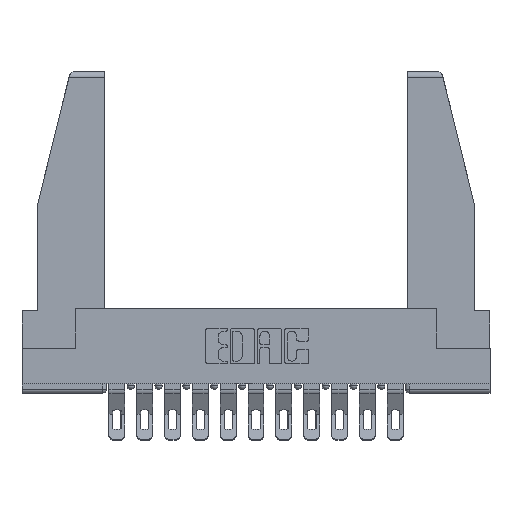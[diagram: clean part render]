
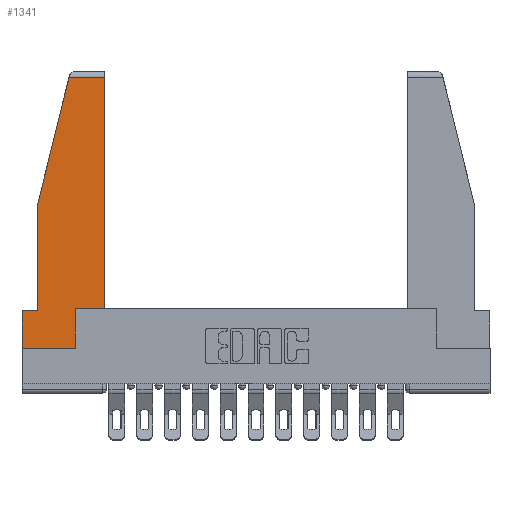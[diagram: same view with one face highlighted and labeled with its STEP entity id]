
A CAD part, top view. The second image highlights one B-rep face of the part: STEP entity #1341.
In plain terms, the highlighted planar face has unit normal (0, 0, 1).
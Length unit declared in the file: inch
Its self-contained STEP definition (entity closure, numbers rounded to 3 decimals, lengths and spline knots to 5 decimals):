
#149 = VERTEX_POINT ( 'NONE', #8627 ) ;
#550 = VERTEX_POINT ( 'NONE', #12458 ) ;
#1341 = ADVANCED_FACE ( 'NONE', ( #1440 ), #10790, .T. ) ;
#1440 = FACE_OUTER_BOUND ( 'NONE', #13769, .T. ) ;
#1858 = DIRECTION ( 'NONE',  ( 0., 0., 1. ) ) ;
#1907 = LINE ( 'NONE', #5243, #12119 ) ;
#2418 = CARTESIAN_POINT ( 'NONE',  ( 0.297, 0., 0. ) ) ;
#3054 = VECTOR ( 'NONE', #14526, 39.37008 ) ;
#3106 = CARTESIAN_POINT ( 'NONE',  ( 0., 0., 0. ) ) ;
#3108 = EDGE_CURVE ( 'NONE', #14425, #3875, #11947, .T. ) ;
#3682 = EDGE_CURVE ( 'NONE', #11848, #14425, #14760, .T. ) ;
#3747 = EDGE_CURVE ( 'NONE', #6221, #11848, #1907, .T. ) ;
#3875 = VERTEX_POINT ( 'NONE', #8193 ) ;
#3944 = EDGE_CURVE ( 'NONE', #13791, #149, #13099, .T. ) ;
#4106 = ORIENTED_EDGE ( 'NONE', *, *, #13910, .T. ) ;
#4577 = CARTESIAN_POINT ( 'NONE',  ( 0.297, 0.223, 0. ) ) ;
#5243 = CARTESIAN_POINT ( 'NONE',  ( 0., 0., 0. ) ) ;
#5554 = LINE ( 'NONE', #12822, #11363 ) ;
#5610 = AXIS2_PLACEMENT_3D ( 'NONE', #3106, #1858, #9544 ) ;
#6158 = VECTOR ( 'NONE', #15853, 39.37008 ) ;
#6221 = VERTEX_POINT ( 'NONE', #10349 ) ;
#6390 = LINE ( 'NONE', #9293, #8972 ) ;
#6427 = CARTESIAN_POINT ( 'NONE',  ( 0.297, 0., 0. ) ) ;
#6461 = ORIENTED_EDGE ( 'NONE', *, *, #3944, .T. ) ;
#6465 = CARTESIAN_POINT ( 'NONE',  ( 0.086, 0.21, 0. ) ) ;
#6560 = VECTOR ( 'NONE', #11701, 39.37008 ) ;
#6715 = VERTEX_POINT ( 'NONE', #11391 ) ;
#7686 = CARTESIAN_POINT ( 'NONE',  ( 0.297, 0.223, 0. ) ) ;
#7864 = DIRECTION ( 'NONE',  ( 1., 0., 0. ) ) ;
#7942 = ORIENTED_EDGE ( 'NONE', *, *, #13602, .T. ) ;
#8193 = CARTESIAN_POINT ( 'NONE',  ( 0.461, 0.223, 0. ) ) ;
#8423 = ORIENTED_EDGE ( 'NONE', *, *, #3682, .T. ) ;
#8551 = EDGE_CURVE ( 'NONE', #149, #550, #5554, .T. ) ;
#8627 = CARTESIAN_POINT ( 'NONE',  ( 0.2636, 1.52, 0. ) ) ;
#8797 = DIRECTION ( 'NONE',  ( 0., 1., 0. ) ) ;
#8857 = DIRECTION ( 'NONE',  ( 1., 0., 0. ) ) ;
#8949 = VECTOR ( 'NONE', #10043, 39.37008 ) ;
#8972 = VECTOR ( 'NONE', #9453, 39.37008 ) ;
#9088 = EDGE_CURVE ( 'NONE', #550, #14053, #11919, .T. ) ;
#9293 = CARTESIAN_POINT ( 'NONE',  ( 0., 0.21, 0. ) ) ;
#9453 = DIRECTION ( 'NONE',  ( -1., 0., 0. ) ) ;
#9478 = CARTESIAN_POINT ( 'NONE',  ( 0., 0.21, 0. ) ) ;
#9544 = DIRECTION ( 'NONE',  ( 1., 0., 0. ) ) ;
#9635 = ORIENTED_EDGE ( 'NONE', *, *, #3108, .T. ) ;
#9905 = CARTESIAN_POINT ( 'NONE',  ( 0.461, 0.223, 0. ) ) ;
#10043 = DIRECTION ( 'NONE',  ( 0., 1., 0. ) ) ;
#10349 = CARTESIAN_POINT ( 'NONE',  ( 0., 0., 0. ) ) ;
#10686 = EDGE_CURVE ( 'NONE', #6715, #6221, #15486, .T. ) ;
#10790 = PLANE ( 'NONE',  #5610 ) ;
#10803 = ORIENTED_EDGE ( 'NONE', *, *, #9088, .T. ) ;
#11363 = VECTOR ( 'NONE', #14133, 39.37008 ) ;
#11391 = CARTESIAN_POINT ( 'NONE',  ( 0., 0.21, 0. ) ) ;
#11571 = VECTOR ( 'NONE', #8857, 39.37008 ) ;
#11701 = DIRECTION ( 'NONE',  ( 0., -1., 0. ) ) ;
#11778 = ORIENTED_EDGE ( 'NONE', *, *, #10686, .T. ) ;
#11848 = VERTEX_POINT ( 'NONE', #6427 ) ;
#11911 = ORIENTED_EDGE ( 'NONE', *, *, #8551, .T. ) ;
#11919 = LINE ( 'NONE', #14325, #6560 ) ;
#11947 = LINE ( 'NONE', #7686, #11571 ) ;
#12119 = VECTOR ( 'NONE', #7864, 39.37008 ) ;
#12458 = CARTESIAN_POINT ( 'NONE',  ( 0.086, 0.8, 0. ) ) ;
#12822 = CARTESIAN_POINT ( 'NONE',  ( 0.271, 1.55, 0. ) ) ;
#13099 = LINE ( 'NONE', #14560, #6158 ) ;
#13337 = VECTOR ( 'NONE', #8797, 39.37008 ) ;
#13602 = EDGE_CURVE ( 'NONE', #14053, #6715, #6390, .T. ) ;
#13769 = EDGE_LOOP ( 'NONE', ( #4106, #6461, #11911, #10803, #7942, #11778, #14488, #8423, #9635 ) ) ;
#13791 = VERTEX_POINT ( 'NONE', #16010 ) ;
#13910 = EDGE_CURVE ( 'NONE', #3875, #13791, #14993, .T. ) ;
#14053 = VERTEX_POINT ( 'NONE', #6465 ) ;
#14133 = DIRECTION ( 'NONE',  ( -0.239, -0.971, 0. ) ) ;
#14325 = CARTESIAN_POINT ( 'NONE',  ( 0.086, 0.8, 0. ) ) ;
#14425 = VERTEX_POINT ( 'NONE', #4577 ) ;
#14488 = ORIENTED_EDGE ( 'NONE', *, *, #3747, .T. ) ;
#14526 = DIRECTION ( 'NONE',  ( 0., -1., 0. ) ) ;
#14560 = CARTESIAN_POINT ( 'NONE',  ( 0., 1.52, 0. ) ) ;
#14760 = LINE ( 'NONE', #2418, #8949 ) ;
#14993 = LINE ( 'NONE', #9905, #13337 ) ;
#15486 = LINE ( 'NONE', #9478, #3054 ) ;
#15853 = DIRECTION ( 'NONE',  ( -1., 0., 0. ) ) ;
#16010 = CARTESIAN_POINT ( 'NONE',  ( 0.461, 1.52, 0. ) ) ;
